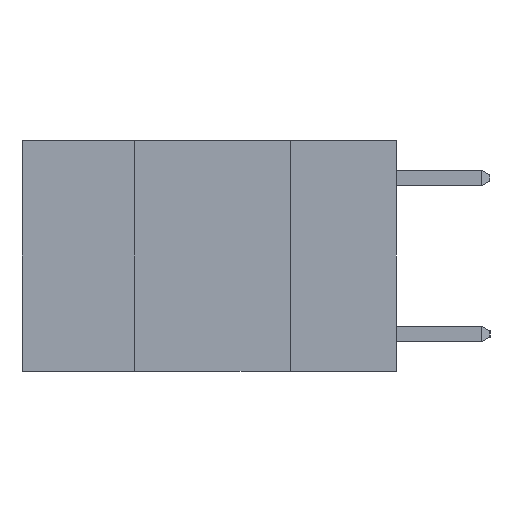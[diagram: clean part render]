
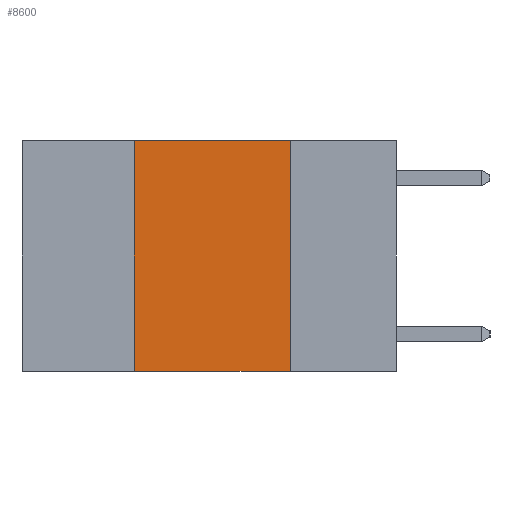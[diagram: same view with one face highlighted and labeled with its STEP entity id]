
A CAD part, left-side view. The second image highlights one B-rep face of the part: STEP entity #8600.
In plain terms, the highlighted planar face has unit normal (-1, 0, 0).
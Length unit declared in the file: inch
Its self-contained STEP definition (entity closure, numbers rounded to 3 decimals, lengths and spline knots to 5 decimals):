
#813 = CARTESIAN_POINT ( 'NONE',  ( 0., 0.42, 0. ) ) ;
#983 = LINE ( 'NONE', #2702, #3273 ) ;
#1807 = CARTESIAN_POINT ( 'NONE',  ( 0., 0.17, 0. ) ) ;
#1987 = VECTOR ( 'NONE', #8738, 39.37008 ) ;
#2043 = LINE ( 'NONE', #1807, #6173 ) ;
#2166 = PLANE ( 'NONE',  #3374 ) ;
#2404 = VERTEX_POINT ( 'NONE', #8386 ) ;
#2702 = CARTESIAN_POINT ( 'NONE',  ( 0., 0.6, -0.37 ) ) ;
#2962 = CARTESIAN_POINT ( 'NONE',  ( 0., 0.6, 0. ) ) ;
#3273 = VECTOR ( 'NONE', #8069, 39.37008 ) ;
#3374 = AXIS2_PLACEMENT_3D ( 'NONE', #2962, #8321, #3759 ) ;
#3737 = VERTEX_POINT ( 'NONE', #813 ) ;
#3759 = DIRECTION ( 'NONE',  ( 0., 0., -1. ) ) ;
#3884 = EDGE_CURVE ( 'NONE', #4445, #2404, #983, .T. ) ;
#4160 = ORIENTED_EDGE ( 'NONE', *, *, #5291, .F. ) ;
#4445 = VERTEX_POINT ( 'NONE', #8670 ) ;
#4939 = ORIENTED_EDGE ( 'NONE', *, *, #6270, .F. ) ;
#5133 = ORIENTED_EDGE ( 'NONE', *, *, #9855, .F. ) ;
#5291 = EDGE_CURVE ( 'NONE', #3737, #7929, #9114, .T. ) ;
#6173 = VECTOR ( 'NONE', #6427, 39.37008 ) ;
#6270 = EDGE_CURVE ( 'NONE', #4445, #3737, #8123, .T. ) ;
#6427 = DIRECTION ( 'NONE',  ( 0., 0., -1. ) ) ;
#6717 = CARTESIAN_POINT ( 'NONE',  ( 0., 0.17, 0. ) ) ;
#7083 = VECTOR ( 'NONE', #7519, 39.37008 ) ;
#7377 = FACE_OUTER_BOUND ( 'NONE', #8098, .T. ) ;
#7519 = DIRECTION ( 'NONE',  ( 0., -1., 0. ) ) ;
#7929 = VERTEX_POINT ( 'NONE', #6717 ) ;
#7957 = CARTESIAN_POINT ( 'NONE',  ( 0., 0.42, 0. ) ) ;
#8069 = DIRECTION ( 'NONE',  ( 0., -1., 0. ) ) ;
#8098 = EDGE_LOOP ( 'NONE', ( #5133, #4160, #4939, #8610 ) ) ;
#8123 = LINE ( 'NONE', #7957, #1987 ) ;
#8321 = DIRECTION ( 'NONE',  ( 1., 0., 0. ) ) ;
#8386 = CARTESIAN_POINT ( 'NONE',  ( 0., 0.17, -0.37 ) ) ;
#8600 = ADVANCED_FACE ( 'NONE', ( #7377 ), #2166, .F. ) ;
#8610 = ORIENTED_EDGE ( 'NONE', *, *, #3884, .T. ) ;
#8670 = CARTESIAN_POINT ( 'NONE',  ( 0., 0.42, -0.37 ) ) ;
#8738 = DIRECTION ( 'NONE',  ( 0., 0., 1. ) ) ;
#9114 = LINE ( 'NONE', #9795, #7083 ) ;
#9795 = CARTESIAN_POINT ( 'NONE',  ( 0., 0.6, 0. ) ) ;
#9855 = EDGE_CURVE ( 'NONE', #7929, #2404, #2043, .T. ) ;
